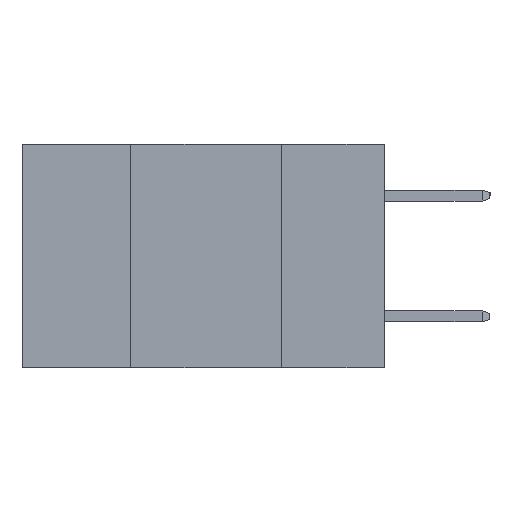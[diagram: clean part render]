
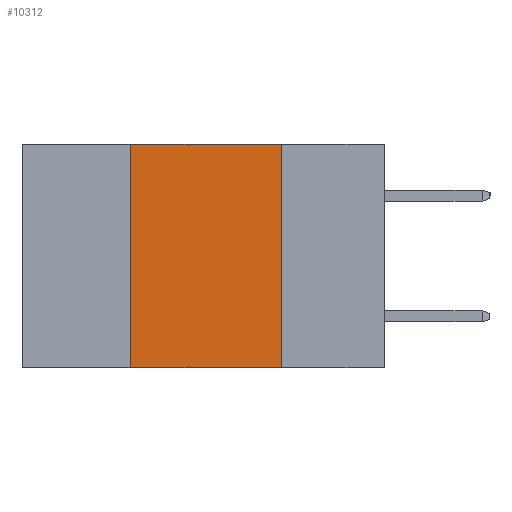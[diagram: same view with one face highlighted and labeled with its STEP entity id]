
A CAD part, left-side view. The second image highlights one B-rep face of the part: STEP entity #10312.
In plain terms, the highlighted planar face has unit normal (-1, 0, 0).
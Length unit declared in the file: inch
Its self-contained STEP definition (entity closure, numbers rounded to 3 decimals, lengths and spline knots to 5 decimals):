
#950 = LINE ( 'NONE', #5935, #8742 ) ;
#964 = EDGE_CURVE ( 'NONE', #3426, #6141, #11651, .T. ) ;
#1066 = EDGE_CURVE ( 'NONE', #5801, #4454, #12295, .T. ) ;
#1517 = CARTESIAN_POINT ( 'NONE',  ( 0., 0.17, -0.37 ) ) ;
#2028 = LINE ( 'NONE', #2268, #3357 ) ;
#2268 = CARTESIAN_POINT ( 'NONE',  ( 0., 0.6, -0.37 ) ) ;
#2663 = EDGE_LOOP ( 'NONE', ( #15970, #9882, #8192, #14879 ) ) ;
#3357 = VECTOR ( 'NONE', #14435, 39.37008 ) ;
#3426 = VERTEX_POINT ( 'NONE', #7507 ) ;
#3789 = CARTESIAN_POINT ( 'NONE',  ( 0., 0.17, -0.37 ) ) ;
#4374 = AXIS2_PLACEMENT_3D ( 'NONE', #14642, #12285, #5915 ) ;
#4454 = VERTEX_POINT ( 'NONE', #1517 ) ;
#5016 = CARTESIAN_POINT ( 'NONE',  ( 0., 0.42, 0. ) ) ;
#5801 = VERTEX_POINT ( 'NONE', #10332 ) ;
#5915 = DIRECTION ( 'NONE',  ( 0., 0., -1. ) ) ;
#5935 = CARTESIAN_POINT ( 'NONE',  ( 0., 0.6, 0. ) ) ;
#6141 = VERTEX_POINT ( 'NONE', #5016 ) ;
#7130 = FACE_OUTER_BOUND ( 'NONE', #2663, .T. ) ;
#7292 = PLANE ( 'NONE',  #4374 ) ;
#7507 = CARTESIAN_POINT ( 'NONE',  ( 0., 0.42, -0.37 ) ) ;
#8192 = ORIENTED_EDGE ( 'NONE', *, *, #964, .F. ) ;
#8587 = EDGE_CURVE ( 'NONE', #6141, #5801, #950, .T. ) ;
#8742 = VECTOR ( 'NONE', #10913, 39.37008 ) ;
#9198 = VECTOR ( 'NONE', #15947, 39.37008 ) ;
#9839 = VECTOR ( 'NONE', #11136, 39.37008 ) ;
#9882 = ORIENTED_EDGE ( 'NONE', *, *, #8587, .F. ) ;
#10312 = ADVANCED_FACE ( 'NONE', ( #7130 ), #7292, .F. ) ;
#10332 = CARTESIAN_POINT ( 'NONE',  ( 0., 0.17, 0. ) ) ;
#10913 = DIRECTION ( 'NONE',  ( 0., -1., 0. ) ) ;
#10983 = CARTESIAN_POINT ( 'NONE',  ( 0., 0.42, -0.37 ) ) ;
#11136 = DIRECTION ( 'NONE',  ( 0., 0., -1. ) ) ;
#11651 = LINE ( 'NONE', #10983, #9198 ) ;
#12285 = DIRECTION ( 'NONE',  ( 1., 0., 0. ) ) ;
#12295 = LINE ( 'NONE', #3789, #9839 ) ;
#13589 = EDGE_CURVE ( 'NONE', #3426, #4454, #2028, .T. ) ;
#14435 = DIRECTION ( 'NONE',  ( 0., -1., 0. ) ) ;
#14642 = CARTESIAN_POINT ( 'NONE',  ( 0., 0.6, 0. ) ) ;
#14879 = ORIENTED_EDGE ( 'NONE', *, *, #13589, .T. ) ;
#15947 = DIRECTION ( 'NONE',  ( 0., 0., 1. ) ) ;
#15970 = ORIENTED_EDGE ( 'NONE', *, *, #1066, .F. ) ;
